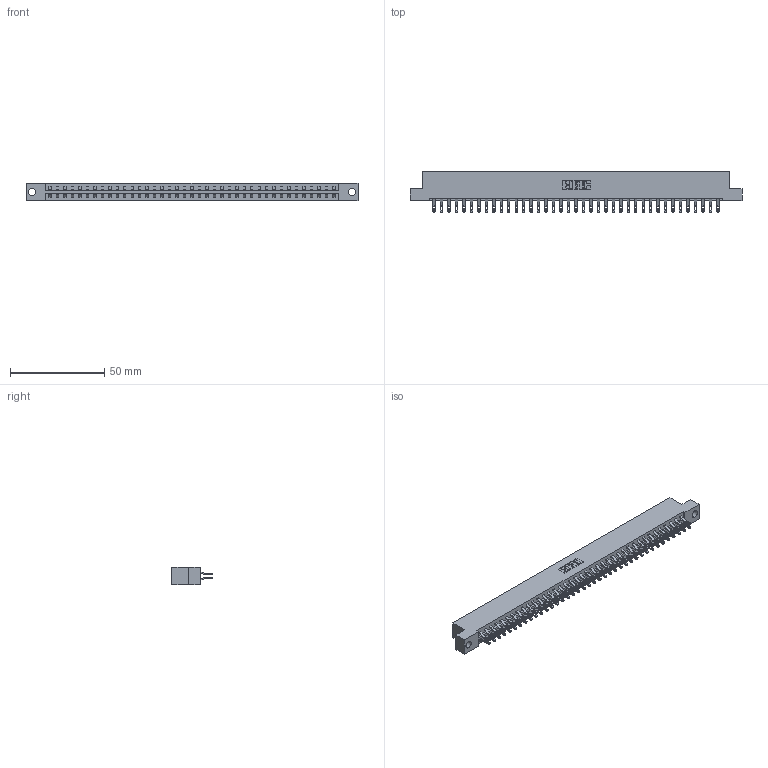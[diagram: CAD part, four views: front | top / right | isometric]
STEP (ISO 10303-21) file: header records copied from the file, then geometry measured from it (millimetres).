
FILE_DESCRIPTION (( 'STEP AP203' ), '1' );
FILE_NAME ('333-078-555-204.STEP', '2018-08-05T00:36:03', ( '' ), ( '' ), 'SwSTEP 2.0', 'SolidWorks 2016', '' );
FILE_SCHEMA (( 'CONFIG_CONTROL_DESIGN' ));
Length unit declared in the file: inch
Products named in the file (3): 333 Part_Flush - .156 Dia - TH; 345-292-001_555 Tail; 333-078-555-204
Assembly tree (79 placements, depth 2):
  333-078-555-204
    333 Part_Flush - .156 Dia - TH
    345-292-001_555 Tail  x78
Bounding box: 176.07 x 21.47 x 9.4 mm (x, y, z)
Volume: 18086.4 mm3; surface area: 21995.9 mm2
Topology: 79 solids, 79 shells, 4638 faces, 14585 edges, 9722 vertices
Faces by surface type: plane 2722, cylinder 1916
Entity records: 25807 total; most frequent: CARTESIAN_POINT 4316, ORIENTED_EDGE 4222, DIRECTION 3663, EDGE_CURVE 2111, LINE 1963, VECTOR 1963, VERTEX_POINT 1406, AXIS2_PLACEMENT_3D 850
